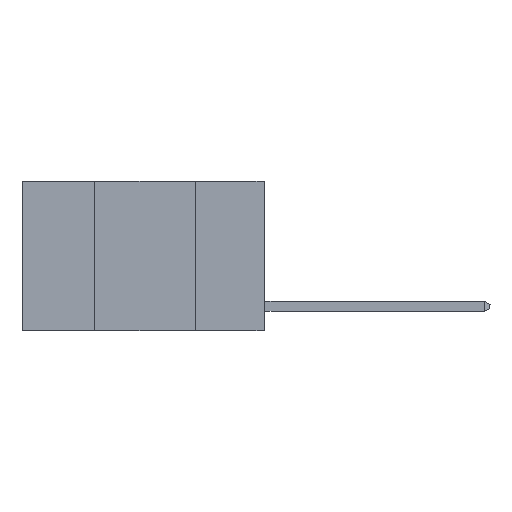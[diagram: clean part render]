
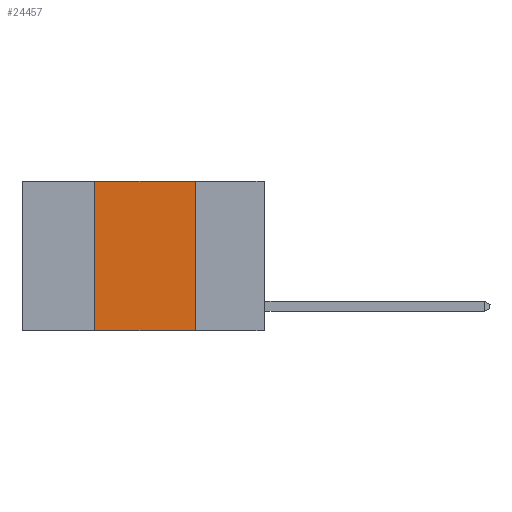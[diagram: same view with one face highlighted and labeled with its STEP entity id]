
A CAD part, left-side view. The second image highlights one B-rep face of the part: STEP entity #24457.
In plain terms, the highlighted planar face has unit normal (-1, 0, 0).
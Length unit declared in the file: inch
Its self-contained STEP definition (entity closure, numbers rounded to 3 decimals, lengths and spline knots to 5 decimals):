
#169 = DIRECTION ( 'NONE',  ( 0., 0., -1. ) ) ;
#1437 = FACE_OUTER_BOUND ( 'NONE', #13861, .T. ) ;
#4108 = ORIENTED_EDGE ( 'NONE', *, *, #7516, .F. ) ;
#4866 = CARTESIAN_POINT ( 'NONE',  ( 0., 0.17, 0. ) ) ;
#5966 = ORIENTED_EDGE ( 'NONE', *, *, #9657, .F. ) ;
#7516 = EDGE_CURVE ( 'NONE', #22801, #8563, #12642, .T. ) ;
#7680 = VECTOR ( 'NONE', #16016, 39.37008 ) ;
#8424 = DIRECTION ( 'NONE',  ( 1., 0., 0. ) ) ;
#8425 = AXIS2_PLACEMENT_3D ( 'NONE', #15279, #8424, #24610 ) ;
#8563 = VERTEX_POINT ( 'NONE', #20048 ) ;
#9657 = EDGE_CURVE ( 'NONE', #23021, #22801, #20566, .T. ) ;
#10581 = EDGE_CURVE ( 'NONE', #17453, #8563, #18809, .T. ) ;
#11031 = CARTESIAN_POINT ( 'NONE',  ( 0., 0.42, 0. ) ) ;
#11921 = VECTOR ( 'NONE', #169, 39.37008 ) ;
#12611 = VECTOR ( 'NONE', #27928, 39.37008 ) ;
#12642 = LINE ( 'NONE', #4866, #11921 ) ;
#12895 = VECTOR ( 'NONE', #20223, 39.37008 ) ;
#13359 = CARTESIAN_POINT ( 'NONE',  ( 0., 0.42, -0.37 ) ) ;
#13666 = CARTESIAN_POINT ( 'NONE',  ( 0., 0.42, 0. ) ) ;
#13861 = EDGE_LOOP ( 'NONE', ( #4108, #5966, #14708, #26269 ) ) ;
#14708 = ORIENTED_EDGE ( 'NONE', *, *, #15645, .F. ) ;
#15279 = CARTESIAN_POINT ( 'NONE',  ( 0., 0.6, 0. ) ) ;
#15645 = EDGE_CURVE ( 'NONE', #17453, #23021, #26094, .T. ) ;
#16016 = DIRECTION ( 'NONE',  ( 0., 0., 1. ) ) ;
#17132 = CARTESIAN_POINT ( 'NONE',  ( 0., 0.17, 0. ) ) ;
#17453 = VERTEX_POINT ( 'NONE', #13359 ) ;
#18809 = LINE ( 'NONE', #25634, #12611 ) ;
#20048 = CARTESIAN_POINT ( 'NONE',  ( 0., 0.17, -0.37 ) ) ;
#20223 = DIRECTION ( 'NONE',  ( 0., -1., 0. ) ) ;
#20566 = LINE ( 'NONE', #29443, #12895 ) ;
#22273 = PLANE ( 'NONE',  #8425 ) ;
#22801 = VERTEX_POINT ( 'NONE', #17132 ) ;
#23021 = VERTEX_POINT ( 'NONE', #11031 ) ;
#24457 = ADVANCED_FACE ( 'NONE', ( #1437 ), #22273, .F. ) ;
#24610 = DIRECTION ( 'NONE',  ( 0., 0., -1. ) ) ;
#25634 = CARTESIAN_POINT ( 'NONE',  ( 0., 0.6, -0.37 ) ) ;
#26094 = LINE ( 'NONE', #13666, #7680 ) ;
#26269 = ORIENTED_EDGE ( 'NONE', *, *, #10581, .T. ) ;
#27928 = DIRECTION ( 'NONE',  ( 0., -1., 0. ) ) ;
#29443 = CARTESIAN_POINT ( 'NONE',  ( 0., 0.6, 0. ) ) ;
